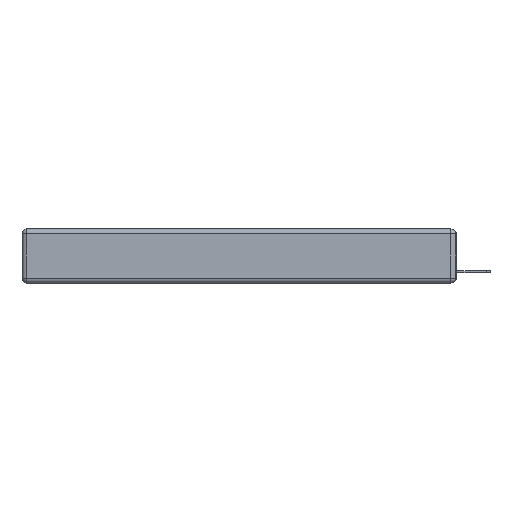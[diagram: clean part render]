
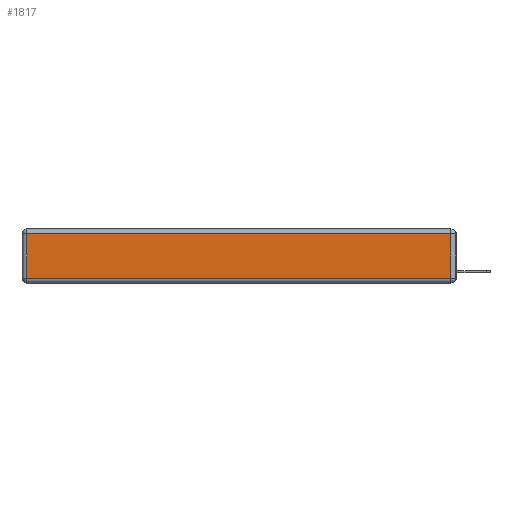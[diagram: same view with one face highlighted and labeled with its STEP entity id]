
A CAD part, left-side view. The second image highlights one B-rep face of the part: STEP entity #1817.
In plain terms, the highlighted planar face has unit normal (-1, 0, 0).
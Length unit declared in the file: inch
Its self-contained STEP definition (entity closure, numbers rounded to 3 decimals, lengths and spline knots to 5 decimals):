
#81 = DIRECTION ( 'NONE',  ( 0., 0., 1. ) ) ;
#473 = LINE ( 'NONE', #671, #6020 ) ;
#671 = CARTESIAN_POINT ( 'NONE',  ( 0., 0., -0.313 ) ) ;
#799 = AXIS2_PLACEMENT_3D ( 'NONE', #2376, #11854, #81 ) ;
#1631 = CARTESIAN_POINT ( 'NONE',  ( 0., 0.03, -0.343 ) ) ;
#1817 = ADVANCED_FACE ( 'NONE', ( #6940 ), #10663, .T. ) ;
#2376 = CARTESIAN_POINT ( 'NONE',  ( 0., 0., -0.343 ) ) ;
#2640 = DIRECTION ( 'NONE',  ( 0., 0., -1. ) ) ;
#3160 = EDGE_CURVE ( 'NONE', #13259, #11665, #5783, .T. ) ;
#3547 = VECTOR ( 'NONE', #14128, 39.37008 ) ;
#3561 = ORIENTED_EDGE ( 'NONE', *, *, #9941, .T. ) ;
#4013 = ORIENTED_EDGE ( 'NONE', *, *, #12225, .T. ) ;
#4330 = DIRECTION ( 'NONE',  ( 0., -1., 0. ) ) ;
#5335 = LINE ( 'NONE', #13229, #14331 ) ;
#5410 = DIRECTION ( 'NONE',  ( 0., 1., 0. ) ) ;
#5783 = LINE ( 'NONE', #1631, #3547 ) ;
#6020 = VECTOR ( 'NONE', #4330, 39.37008 ) ;
#6207 = ORIENTED_EDGE ( 'NONE', *, *, #3160, .T. ) ;
#6777 = VERTEX_POINT ( 'NONE', #15257 ) ;
#6940 = FACE_OUTER_BOUND ( 'NONE', #9824, .T. ) ;
#9214 = ORIENTED_EDGE ( 'NONE', *, *, #15064, .T. ) ;
#9337 = CARTESIAN_POINT ( 'NONE',  ( 0., 2.72, -0.03 ) ) ;
#9824 = EDGE_LOOP ( 'NONE', ( #4013, #6207, #9214, #3561 ) ) ;
#9941 = EDGE_CURVE ( 'NONE', #10607, #6777, #5335, .T. ) ;
#10107 = CARTESIAN_POINT ( 'NONE',  ( 0., 2.75, -0.03 ) ) ;
#10607 = VERTEX_POINT ( 'NONE', #9337 ) ;
#10663 = PLANE ( 'NONE',  #799 ) ;
#10847 = CARTESIAN_POINT ( 'NONE',  ( 0., 0.03, -0.313 ) ) ;
#11665 = VERTEX_POINT ( 'NONE', #12329 ) ;
#11854 = DIRECTION ( 'NONE',  ( -1., 0., 0. ) ) ;
#12225 = EDGE_CURVE ( 'NONE', #6777, #13259, #473, .T. ) ;
#12247 = VECTOR ( 'NONE', #5410, 39.37008 ) ;
#12329 = CARTESIAN_POINT ( 'NONE',  ( 0., 0.03, -0.03 ) ) ;
#13229 = CARTESIAN_POINT ( 'NONE',  ( 0., 2.72, -0.343 ) ) ;
#13259 = VERTEX_POINT ( 'NONE', #10847 ) ;
#14128 = DIRECTION ( 'NONE',  ( 0., 0., 1. ) ) ;
#14331 = VECTOR ( 'NONE', #2640, 39.37008 ) ;
#14440 = LINE ( 'NONE', #10107, #12247 ) ;
#15064 = EDGE_CURVE ( 'NONE', #11665, #10607, #14440, .T. ) ;
#15257 = CARTESIAN_POINT ( 'NONE',  ( 0., 2.72, -0.313 ) ) ;
